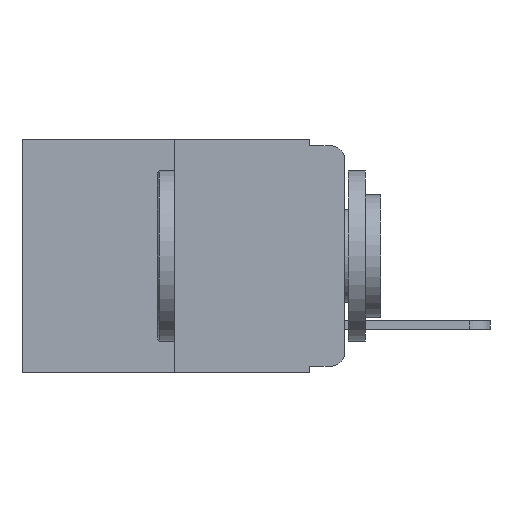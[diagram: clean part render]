
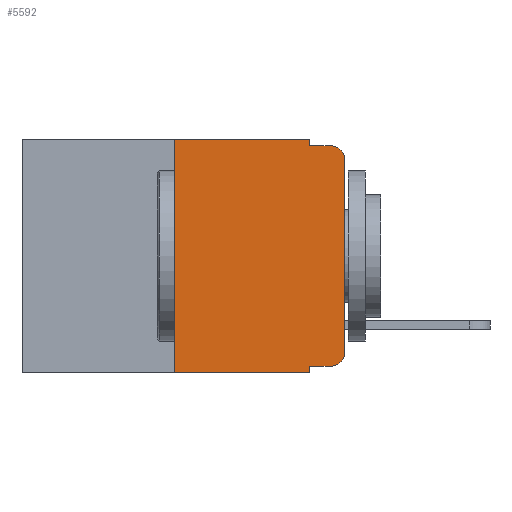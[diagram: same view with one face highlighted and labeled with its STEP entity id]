
A CAD part, left-side view. The second image highlights one B-rep face of the part: STEP entity #5592.
In plain terms, the highlighted planar face has unit normal (-1, 0, 0).
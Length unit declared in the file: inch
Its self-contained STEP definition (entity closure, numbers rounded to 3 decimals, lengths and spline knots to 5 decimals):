
#361 = CARTESIAN_POINT ( 'NONE',  ( 0., 0.051, -0.01 ) ) ;
#456 = DIRECTION ( 'NONE',  ( -1., 0., 0. ) ) ;
#1390 = VECTOR ( 'NONE', #10349, 39.37008 ) ;
#1790 = EDGE_CURVE ( 'NONE', #2287, #13399, #21267, .T. ) ;
#2096 = ORIENTED_EDGE ( 'NONE', *, *, #12740, .F. ) ;
#2287 = VERTEX_POINT ( 'NONE', #20801 ) ;
#2640 = ORIENTED_EDGE ( 'NONE', *, *, #14519, .T. ) ;
#2911 = DIRECTION ( 'NONE',  ( 0., 0., -1. ) ) ;
#3002 = CARTESIAN_POINT ( 'NONE',  ( 0., 0.02, -0.01 ) ) ;
#3003 = EDGE_CURVE ( 'NONE', #19976, #12321, #12330, .T. ) ;
#3040 = ORIENTED_EDGE ( 'NONE', *, *, #14159, .T. ) ;
#3079 = CARTESIAN_POINT ( 'NONE',  ( 0., 0.051, 0. ) ) ;
#3229 = VECTOR ( 'NONE', #23537, 39.37008 ) ;
#3584 = ORIENTED_EDGE ( 'NONE', *, *, #4140, .F. ) ;
#4043 = VECTOR ( 'NONE', #9219, 39.37008 ) ;
#4108 = EDGE_CURVE ( 'NONE', #9017, #8933, #14763, .T. ) ;
#4140 = EDGE_CURVE ( 'NONE', #24105, #13399, #11492, .T. ) ;
#4705 = EDGE_CURVE ( 'NONE', #15429, #9017, #14114, .T. ) ;
#5554 = DIRECTION ( 'NONE',  ( 0., 0., -1. ) ) ;
#5565 = CARTESIAN_POINT ( 'NONE',  ( 0., 0.051, -0.333 ) ) ;
#5592 = ADVANCED_FACE ( 'NONE', ( #16753 ), #20040, .F. ) ;
#5769 = ORIENTED_EDGE ( 'NONE', *, *, #4705, .F. ) ;
#5844 = LINE ( 'NONE', #16868, #20624 ) ;
#5872 = ORIENTED_EDGE ( 'NONE', *, *, #3003, .T. ) ;
#6665 = ORIENTED_EDGE ( 'NONE', *, *, #15572, .T. ) ;
#7636 = CARTESIAN_POINT ( 'NONE',  ( 0., 0.25, 0. ) ) ;
#7867 = VERTEX_POINT ( 'NONE', #17550 ) ;
#7887 = VERTEX_POINT ( 'NONE', #15345 ) ;
#8353 = CARTESIAN_POINT ( 'NONE',  ( 0., 0., 0. ) ) ;
#8933 = VERTEX_POINT ( 'NONE', #12732 ) ;
#9017 = VERTEX_POINT ( 'NONE', #7636 ) ;
#9138 = LINE ( 'NONE', #13669, #13008 ) ;
#9165 = CARTESIAN_POINT ( 'NONE',  ( 0., 0.02, -0.03 ) ) ;
#9219 = DIRECTION ( 'NONE',  ( 0., 0., 1. ) ) ;
#9402 = EDGE_LOOP ( 'NONE', ( #3040, #16584, #3584, #17715, #10165, #5769, #2640, #2096, #5872, #6665 ) ) ;
#9729 = VECTOR ( 'NONE', #17722, 39.37008 ) ;
#10165 = ORIENTED_EDGE ( 'NONE', *, *, #4108, .F. ) ;
#10289 = CARTESIAN_POINT ( 'NONE',  ( 0., 0.473, 0. ) ) ;
#10349 = DIRECTION ( 'NONE',  ( 0., -1., 0. ) ) ;
#10615 = DIRECTION ( 'NONE',  ( 1., 0., 0. ) ) ;
#10978 = DIRECTION ( 'NONE',  ( -1., 0., 0. ) ) ;
#11055 = AXIS2_PLACEMENT_3D ( 'NONE', #9165, #10978, #24516 ) ;
#11492 = LINE ( 'NONE', #21667, #1390 ) ;
#12079 = CARTESIAN_POINT ( 'NONE',  ( 0., 0.473, 0. ) ) ;
#12321 = VERTEX_POINT ( 'NONE', #16917 ) ;
#12330 = LINE ( 'NONE', #5565, #19431 ) ;
#12732 = CARTESIAN_POINT ( 'NONE',  ( 0., 0.051, 0. ) ) ;
#12740 = EDGE_CURVE ( 'NONE', #19976, #7867, #9138, .T. ) ;
#13008 = VECTOR ( 'NONE', #19134, 39.37008 ) ;
#13113 = DIRECTION ( 'NONE',  ( 0., -1., 0. ) ) ;
#13167 = EDGE_CURVE ( 'NONE', #8933, #24105, #21585, .T. ) ;
#13297 = LINE ( 'NONE', #8353, #21823 ) ;
#13399 = VERTEX_POINT ( 'NONE', #3002 ) ;
#13669 = CARTESIAN_POINT ( 'NONE',  ( 0., 0.051, 0. ) ) ;
#14114 = LINE ( 'NONE', #20539, #4043 ) ;
#14159 = EDGE_CURVE ( 'NONE', #7887, #2287, #13297, .T. ) ;
#14519 = EDGE_CURVE ( 'NONE', #15429, #7867, #5844, .T. ) ;
#14763 = LINE ( 'NONE', #12079, #9729 ) ;
#15199 = DIRECTION ( 'NONE',  ( 0., -1., 0. ) ) ;
#15345 = CARTESIAN_POINT ( 'NONE',  ( 0., 0., -0.313 ) ) ;
#15429 = VERTEX_POINT ( 'NONE', #16012 ) ;
#15572 = EDGE_CURVE ( 'NONE', #12321, #7887, #16630, .T. ) ;
#16012 = CARTESIAN_POINT ( 'NONE',  ( 0., 0.25, -0.343 ) ) ;
#16584 = ORIENTED_EDGE ( 'NONE', *, *, #1790, .T. ) ;
#16630 = CIRCLE ( 'NONE', #23514, 0.02 ) ;
#16753 = FACE_OUTER_BOUND ( 'NONE', #9402, .T. ) ;
#16868 = CARTESIAN_POINT ( 'NONE',  ( 0., 0.473, -0.343 ) ) ;
#16917 = CARTESIAN_POINT ( 'NONE',  ( 0., 0.02, -0.333 ) ) ;
#17550 = CARTESIAN_POINT ( 'NONE',  ( 0., 0.051, -0.343 ) ) ;
#17715 = ORIENTED_EDGE ( 'NONE', *, *, #13167, .F. ) ;
#17722 = DIRECTION ( 'NONE',  ( 0., -1., 0. ) ) ;
#19134 = DIRECTION ( 'NONE',  ( 0., 0., -1. ) ) ;
#19431 = VECTOR ( 'NONE', #13113, 39.37008 ) ;
#19476 = DIRECTION ( 'NONE',  ( 0., 0., 1. ) ) ;
#19976 = VERTEX_POINT ( 'NONE', #23692 ) ;
#20040 = PLANE ( 'NONE',  #21227 ) ;
#20508 = CARTESIAN_POINT ( 'NONE',  ( 0., 0.02, -0.313 ) ) ;
#20539 = CARTESIAN_POINT ( 'NONE',  ( 0., 0.25, 0. ) ) ;
#20624 = VECTOR ( 'NONE', #15199, 39.37008 ) ;
#20801 = CARTESIAN_POINT ( 'NONE',  ( 0., 0., -0.03 ) ) ;
#21227 = AXIS2_PLACEMENT_3D ( 'NONE', #10289, #10615, #2911 ) ;
#21267 = CIRCLE ( 'NONE', #11055, 0.02 ) ;
#21585 = LINE ( 'NONE', #3079, #3229 ) ;
#21667 = CARTESIAN_POINT ( 'NONE',  ( 0., 0.051, -0.01 ) ) ;
#21823 = VECTOR ( 'NONE', #19476, 39.37008 ) ;
#23514 = AXIS2_PLACEMENT_3D ( 'NONE', #20508, #456, #5554 ) ;
#23537 = DIRECTION ( 'NONE',  ( 0., 0., -1. ) ) ;
#23692 = CARTESIAN_POINT ( 'NONE',  ( 0., 0.051, -0.333 ) ) ;
#24105 = VERTEX_POINT ( 'NONE', #361 ) ;
#24516 = DIRECTION ( 'NONE',  ( 0., 0., -1. ) ) ;
